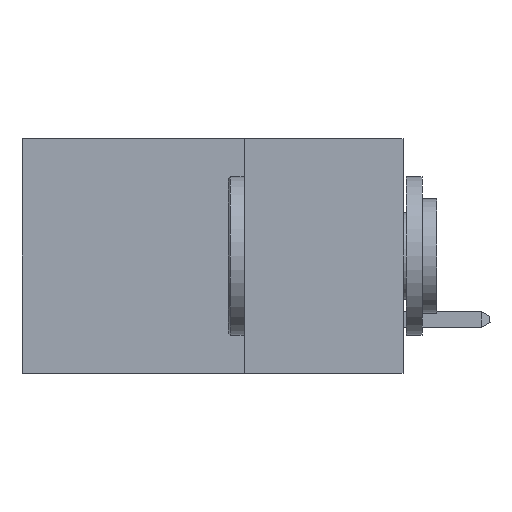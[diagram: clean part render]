
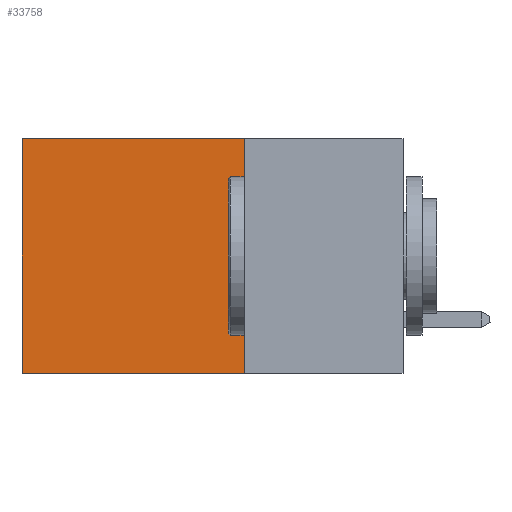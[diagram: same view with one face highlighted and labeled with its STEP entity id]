
A CAD part, left-side view. The second image highlights one B-rep face of the part: STEP entity #33758.
In plain terms, the highlighted planar face has unit normal (-1, 0, 0).
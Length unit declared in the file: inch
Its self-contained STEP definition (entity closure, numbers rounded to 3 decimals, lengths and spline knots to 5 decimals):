
#93 = CARTESIAN_POINT ( 'NONE',  ( 0.2875, 0.25, -0.37 ) ) ;
#1225 = ORIENTED_EDGE ( 'NONE', *, *, #20198, .F. ) ;
#1855 = VERTEX_POINT ( 'NONE', #93 ) ;
#2123 = DIRECTION ( 'NONE',  ( 0., 0., -1. ) ) ;
#3008 = CARTESIAN_POINT ( 'NONE',  ( 0.2875, 0.6, -0.37 ) ) ;
#4784 = DIRECTION ( 'NONE',  ( 0., 0., -1. ) ) ;
#6068 = DIRECTION ( 'NONE',  ( 0., 1., 0. ) ) ;
#6953 = CARTESIAN_POINT ( 'NONE',  ( 0.2875, 0.25, -0.37 ) ) ;
#8124 = PLANE ( 'NONE',  #24230 ) ;
#8307 = VECTOR ( 'NONE', #2123, 39.37008 ) ;
#12101 = VECTOR ( 'NONE', #18569, 39.37008 ) ;
#13723 = ORIENTED_EDGE ( 'NONE', *, *, #31354, .T. ) ;
#14272 = EDGE_CURVE ( 'NONE', #20238, #40458, #42468, .T. ) ;
#17350 = VECTOR ( 'NONE', #6068, 39.37008 ) ;
#17444 = CARTESIAN_POINT ( 'NONE',  ( 0.2875, 0.6, 0. ) ) ;
#18569 = DIRECTION ( 'NONE',  ( 0., 1., 0. ) ) ;
#19707 = ORIENTED_EDGE ( 'NONE', *, *, #14272, .T. ) ;
#20198 = EDGE_CURVE ( 'NONE', #1855, #40458, #23407, .T. ) ;
#20238 = VERTEX_POINT ( 'NONE', #37537 ) ;
#20390 = DIRECTION ( 'NONE',  ( 0., 0., -1. ) ) ;
#23407 = LINE ( 'NONE', #6953, #12101 ) ;
#24230 = AXIS2_PLACEMENT_3D ( 'NONE', #27821, #42940, #4784 ) ;
#24371 = CARTESIAN_POINT ( 'NONE',  ( 0.2875, 0.25, 0. ) ) ;
#26063 = FACE_OUTER_BOUND ( 'NONE', #41425, .T. ) ;
#27821 = CARTESIAN_POINT ( 'NONE',  ( 0.2875, 0.25, 0. ) ) ;
#30556 = LINE ( 'NONE', #24371, #17350 ) ;
#30713 = LINE ( 'NONE', #32104, #38518 ) ;
#31354 = EDGE_CURVE ( 'NONE', #46290, #20238, #30556, .T. ) ;
#32104 = CARTESIAN_POINT ( 'NONE',  ( 0.2875, 0.25, 0. ) ) ;
#33758 = ADVANCED_FACE ( 'NONE', ( #26063 ), #8124, .F. ) ;
#34598 = EDGE_CURVE ( 'NONE', #46290, #1855, #30713, .T. ) ;
#35467 = ORIENTED_EDGE ( 'NONE', *, *, #34598, .F. ) ;
#37537 = CARTESIAN_POINT ( 'NONE',  ( 0.2875, 0.6, 0. ) ) ;
#38518 = VECTOR ( 'NONE', #20390, 39.37008 ) ;
#40458 = VERTEX_POINT ( 'NONE', #3008 ) ;
#41425 = EDGE_LOOP ( 'NONE', ( #19707, #1225, #35467, #13723 ) ) ;
#42468 = LINE ( 'NONE', #17444, #8307 ) ;
#42940 = DIRECTION ( 'NONE',  ( 1., 0., 0. ) ) ;
#46290 = VERTEX_POINT ( 'NONE', #46712 ) ;
#46712 = CARTESIAN_POINT ( 'NONE',  ( 0.2875, 0.25, 0. ) ) ;
